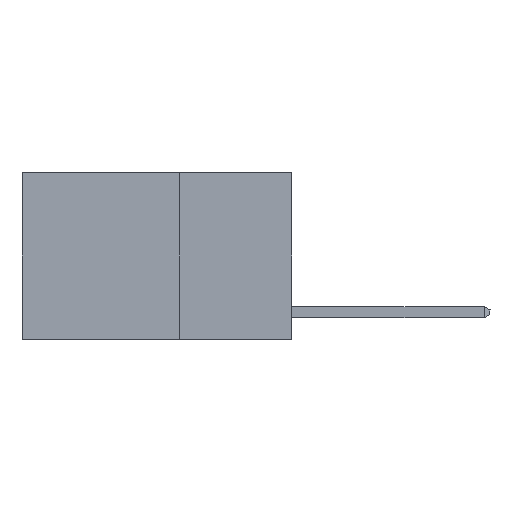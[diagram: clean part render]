
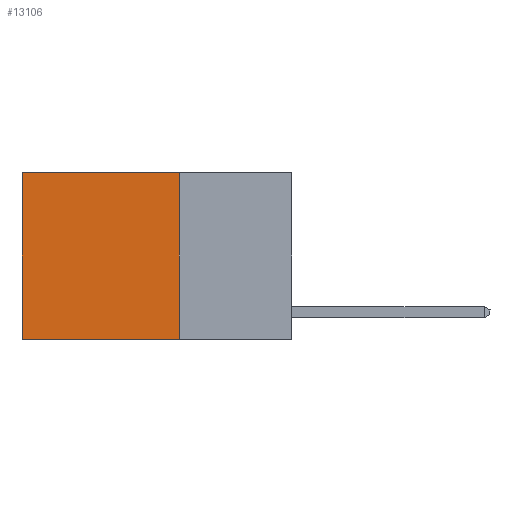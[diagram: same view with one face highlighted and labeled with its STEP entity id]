
A CAD part, left-side view. The second image highlights one B-rep face of the part: STEP entity #13106.
In plain terms, the highlighted planar face has unit normal (-1, 0, 0).
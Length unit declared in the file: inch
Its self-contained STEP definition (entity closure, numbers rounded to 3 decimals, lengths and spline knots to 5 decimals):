
#300 = DIRECTION ( 'NONE',  ( 0., 1., 0. ) ) ;
#369 = CARTESIAN_POINT ( 'NONE',  ( 0.2625, 0.6, 0. ) ) ;
#542 = CARTESIAN_POINT ( 'NONE',  ( 0.2625, 0.25, -0.37 ) ) ;
#971 = ORIENTED_EDGE ( 'NONE', *, *, #10016, .F. ) ;
#1428 = DIRECTION ( 'NONE',  ( 0., 0., -1. ) ) ;
#2612 = DIRECTION ( 'NONE',  ( 0., 0., -1. ) ) ;
#4605 = VECTOR ( 'NONE', #2612, 39.37008 ) ;
#5186 = VECTOR ( 'NONE', #300, 39.37008 ) ;
#5284 = ORIENTED_EDGE ( 'NONE', *, *, #18809, .T. ) ;
#5802 = PLANE ( 'NONE',  #11699 ) ;
#5860 = ORIENTED_EDGE ( 'NONE', *, *, #11770, .F. ) ;
#6143 = ORIENTED_EDGE ( 'NONE', *, *, #23154, .T. ) ;
#7232 = EDGE_LOOP ( 'NONE', ( #6143, #971, #5860, #5284 ) ) ;
#7693 = CARTESIAN_POINT ( 'NONE',  ( 0.2625, 0.25, -0.37 ) ) ;
#8028 = CARTESIAN_POINT ( 'NONE',  ( 0.2625, 0.25, 0. ) ) ;
#8595 = VECTOR ( 'NONE', #10276, 39.37008 ) ;
#9925 = DIRECTION ( 'NONE',  ( 0., 1., 0. ) ) ;
#10016 = EDGE_CURVE ( 'NONE', #16048, #28006, #20175, .T. ) ;
#10276 = DIRECTION ( 'NONE',  ( 0., 0., -1. ) ) ;
#10494 = VERTEX_POINT ( 'NONE', #20814 ) ;
#10547 = LINE ( 'NONE', #369, #4605 ) ;
#11699 = AXIS2_PLACEMENT_3D ( 'NONE', #28247, #14800, #1428 ) ;
#11770 = EDGE_CURVE ( 'NONE', #22114, #16048, #26487, .T. ) ;
#13106 = ADVANCED_FACE ( 'NONE', ( #25020 ), #5802, .F. ) ;
#14800 = DIRECTION ( 'NONE',  ( 1., 0., 0. ) ) ;
#15955 = CARTESIAN_POINT ( 'NONE',  ( 0.2625, 0.25, 0. ) ) ;
#16048 = VERTEX_POINT ( 'NONE', #542 ) ;
#17416 = CARTESIAN_POINT ( 'NONE',  ( 0.2625, 0.6, -0.37 ) ) ;
#18528 = LINE ( 'NONE', #15955, #5186 ) ;
#18763 = VECTOR ( 'NONE', #9925, 39.37008 ) ;
#18809 = EDGE_CURVE ( 'NONE', #22114, #10494, #18528, .T. ) ;
#20175 = LINE ( 'NONE', #7693, #18763 ) ;
#20814 = CARTESIAN_POINT ( 'NONE',  ( 0.2625, 0.6, 0. ) ) ;
#22114 = VERTEX_POINT ( 'NONE', #26727 ) ;
#23154 = EDGE_CURVE ( 'NONE', #10494, #28006, #10547, .T. ) ;
#25020 = FACE_OUTER_BOUND ( 'NONE', #7232, .T. ) ;
#26487 = LINE ( 'NONE', #8028, #8595 ) ;
#26727 = CARTESIAN_POINT ( 'NONE',  ( 0.2625, 0.25, 0. ) ) ;
#28006 = VERTEX_POINT ( 'NONE', #17416 ) ;
#28247 = CARTESIAN_POINT ( 'NONE',  ( 0.2625, 0.25, 0. ) ) ;
